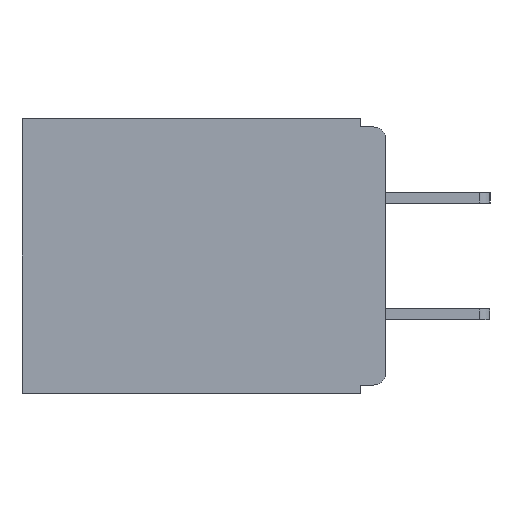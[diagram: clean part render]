
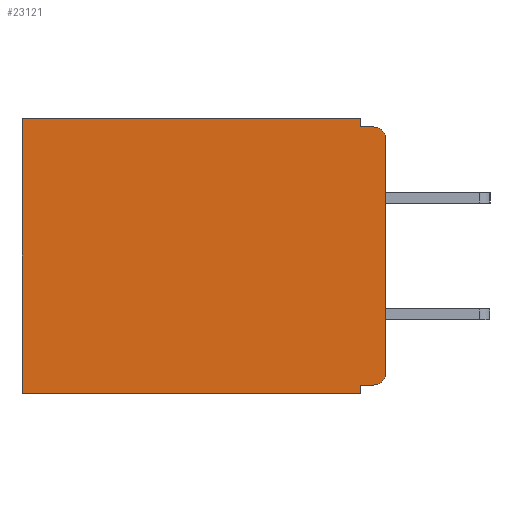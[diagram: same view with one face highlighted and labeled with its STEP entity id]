
A CAD part, left-side view. The second image highlights one B-rep face of the part: STEP entity #23121.
In plain terms, the highlighted planar face has unit normal (-1, 0, 0).
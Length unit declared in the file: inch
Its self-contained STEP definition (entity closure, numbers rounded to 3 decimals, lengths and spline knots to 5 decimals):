
#717 = ORIENTED_EDGE ( 'NONE', *, *, #9996, .T. ) ;
#732 = DIRECTION ( 'NONE',  ( 0., 1., 0. ) ) ;
#1000 = CARTESIAN_POINT ( 'NONE',  ( 0.3, 0.437, -0.33 ) ) ;
#1015 = EDGE_CURVE ( 'NONE', #4376, #20245, #17150, .T. ) ;
#1495 = LINE ( 'NONE', #31475, #21164 ) ;
#1867 = CARTESIAN_POINT ( 'NONE',  ( 0.3, 0., -0.305 ) ) ;
#2744 = CARTESIAN_POINT ( 'NONE',  ( 0.3, 0.031, -0.33 ) ) ;
#2872 = ORIENTED_EDGE ( 'NONE', *, *, #19030, .F. ) ;
#3629 = AXIS2_PLACEMENT_3D ( 'NONE', #11492, #11464, #11306 ) ;
#4127 = VERTEX_POINT ( 'NONE', #22629 ) ;
#4376 = VERTEX_POINT ( 'NONE', #12819 ) ;
#4802 = VERTEX_POINT ( 'NONE', #20045 ) ;
#4905 = DIRECTION ( 'NONE',  ( 0., 0., -1. ) ) ;
#5421 = ORIENTED_EDGE ( 'NONE', *, *, #31270, .F. ) ;
#5771 = LINE ( 'NONE', #25314, #12099 ) ;
#6134 = EDGE_CURVE ( 'NONE', #12453, #24401, #30187, .T. ) ;
#6473 = CARTESIAN_POINT ( 'NONE',  ( 0.3, 0.437, -0.33 ) ) ;
#6614 = DIRECTION ( 'NONE',  ( 0., 1., 0. ) ) ;
#7366 = FACE_OUTER_BOUND ( 'NONE', #18434, .T. ) ;
#7527 = EDGE_CURVE ( 'NONE', #18693, #9541, #22259, .T. ) ;
#7779 = DIRECTION ( 'NONE',  ( 0., 0., -1. ) ) ;
#7884 = ORIENTED_EDGE ( 'NONE', *, *, #1015, .F. ) ;
#8499 = DIRECTION ( 'NONE',  ( 0., 0., -1. ) ) ;
#8960 = VECTOR ( 'NONE', #6614, 39.37008 ) ;
#9541 = VERTEX_POINT ( 'NONE', #6473 ) ;
#9996 = EDGE_CURVE ( 'NONE', #4802, #26758, #18829, .T. ) ;
#11306 = DIRECTION ( 'NONE',  ( 0., 0., -1. ) ) ;
#11464 = DIRECTION ( 'NONE',  ( -1., 0., 0. ) ) ;
#11492 = CARTESIAN_POINT ( 'NONE',  ( 0.3, 0.015, -0.305 ) ) ;
#11515 = DIRECTION ( 'NONE',  ( -1., 0., 0. ) ) ;
#12099 = VECTOR ( 'NONE', #27984, 39.37008 ) ;
#12453 = VERTEX_POINT ( 'NONE', #16134 ) ;
#12819 = CARTESIAN_POINT ( 'NONE',  ( 0.3, 0.031, 0. ) ) ;
#12952 = AXIS2_PLACEMENT_3D ( 'NONE', #27451, #11515, #30037 ) ;
#12953 = LINE ( 'NONE', #29830, #33126 ) ;
#13012 = LINE ( 'NONE', #13323, #27171 ) ;
#13323 = CARTESIAN_POINT ( 'NONE',  ( 0.3, 0., -0.33 ) ) ;
#15139 = CARTESIAN_POINT ( 'NONE',  ( 0.3, 0.031, -0.01 ) ) ;
#15212 = PLANE ( 'NONE',  #25723 ) ;
#16134 = CARTESIAN_POINT ( 'NONE',  ( 0.3, 0.015, -0.32 ) ) ;
#17150 = LINE ( 'NONE', #30589, #23342 ) ;
#17938 = DIRECTION ( 'NONE',  ( 0., 0., -1. ) ) ;
#18213 = EDGE_CURVE ( 'NONE', #4802, #24401, #13012, .T. ) ;
#18254 = VERTEX_POINT ( 'NONE', #2744 ) ;
#18434 = EDGE_LOOP ( 'NONE', ( #18799, #717, #26676, #7884, #29947, #30360, #2872, #5421, #32355, #27991 ) ) ;
#18693 = VERTEX_POINT ( 'NONE', #31071 ) ;
#18799 = ORIENTED_EDGE ( 'NONE', *, *, #18213, .F. ) ;
#18829 = CIRCLE ( 'NONE', #12952, 0.015 ) ;
#19030 = EDGE_CURVE ( 'NONE', #18254, #9541, #12953, .T. ) ;
#19353 = VECTOR ( 'NONE', #732, 39.37008 ) ;
#20045 = CARTESIAN_POINT ( 'NONE',  ( 0.3, 0., -0.025 ) ) ;
#20245 = VERTEX_POINT ( 'NONE', #15139 ) ;
#20942 = DIRECTION ( 'NONE',  ( 0., 0., -1. ) ) ;
#21164 = VECTOR ( 'NONE', #20942, 39.37008 ) ;
#22142 = CARTESIAN_POINT ( 'NONE',  ( 0.3, 0., 0. ) ) ;
#22259 = LINE ( 'NONE', #1000, #28486 ) ;
#22629 = CARTESIAN_POINT ( 'NONE',  ( 0.3, 0.031, -0.32 ) ) ;
#22702 = CARTESIAN_POINT ( 'NONE',  ( 0.3, 0., -0.32 ) ) ;
#23121 = ADVANCED_FACE ( 'NONE', ( #7366 ), #15212, .F. ) ;
#23342 = VECTOR ( 'NONE', #4905, 39.37008 ) ;
#24401 = VERTEX_POINT ( 'NONE', #1867 ) ;
#24551 = DIRECTION ( 'NONE',  ( 0., 1., 0. ) ) ;
#25314 = CARTESIAN_POINT ( 'NONE',  ( 0.3, 0., -0.01 ) ) ;
#25723 = AXIS2_PLACEMENT_3D ( 'NONE', #31005, #33576, #17938 ) ;
#26676 = ORIENTED_EDGE ( 'NONE', *, *, #30239, .F. ) ;
#26758 = VERTEX_POINT ( 'NONE', #33991 ) ;
#27171 = VECTOR ( 'NONE', #7779, 39.37008 ) ;
#27451 = CARTESIAN_POINT ( 'NONE',  ( 0.3, 0.015, -0.025 ) ) ;
#27739 = LINE ( 'NONE', #22702, #8960 ) ;
#27984 = DIRECTION ( 'NONE',  ( 0., -1., 0. ) ) ;
#27991 = ORIENTED_EDGE ( 'NONE', *, *, #6134, .T. ) ;
#28486 = VECTOR ( 'NONE', #8499, 39.37008 ) ;
#29830 = CARTESIAN_POINT ( 'NONE',  ( 0.3, 0., -0.33 ) ) ;
#29947 = ORIENTED_EDGE ( 'NONE', *, *, #33838, .T. ) ;
#30037 = DIRECTION ( 'NONE',  ( 0., 0., -1. ) ) ;
#30187 = CIRCLE ( 'NONE', #3629, 0.015 ) ;
#30239 = EDGE_CURVE ( 'NONE', #20245, #26758, #5771, .T. ) ;
#30360 = ORIENTED_EDGE ( 'NONE', *, *, #7527, .T. ) ;
#30589 = CARTESIAN_POINT ( 'NONE',  ( 0.3, 0.031, 0. ) ) ;
#31005 = CARTESIAN_POINT ( 'NONE',  ( 0.3, 0., -0.33 ) ) ;
#31071 = CARTESIAN_POINT ( 'NONE',  ( 0.3, 0.437, 0. ) ) ;
#31270 = EDGE_CURVE ( 'NONE', #4127, #18254, #1495, .T. ) ;
#31475 = CARTESIAN_POINT ( 'NONE',  ( 0.3, 0.031, -0.33 ) ) ;
#32276 = EDGE_CURVE ( 'NONE', #12453, #4127, #27739, .T. ) ;
#32355 = ORIENTED_EDGE ( 'NONE', *, *, #32276, .F. ) ;
#33126 = VECTOR ( 'NONE', #24551, 39.37008 ) ;
#33218 = LINE ( 'NONE', #22142, #19353 ) ;
#33576 = DIRECTION ( 'NONE',  ( 1., 0., 0. ) ) ;
#33838 = EDGE_CURVE ( 'NONE', #4376, #18693, #33218, .T. ) ;
#33991 = CARTESIAN_POINT ( 'NONE',  ( 0.3, 0.015, -0.01 ) ) ;
